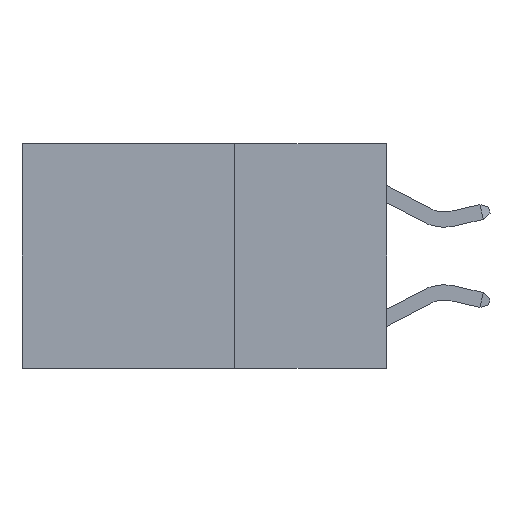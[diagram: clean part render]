
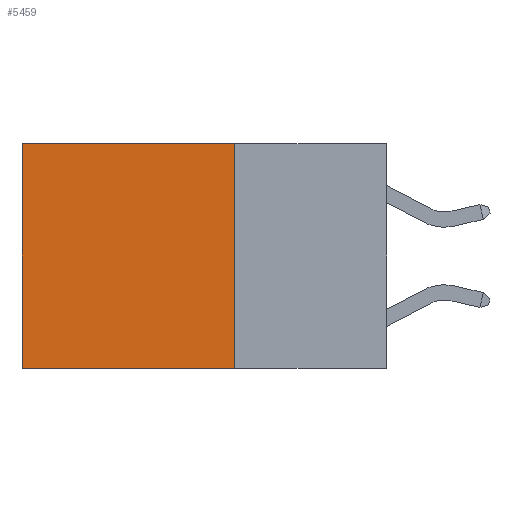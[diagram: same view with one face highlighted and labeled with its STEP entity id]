
A CAD part, left-side view. The second image highlights one B-rep face of the part: STEP entity #5459.
In plain terms, the highlighted planar face has unit normal (-1, 0, 0).
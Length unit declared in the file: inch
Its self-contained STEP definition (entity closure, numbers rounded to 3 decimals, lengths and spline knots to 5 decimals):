
#92 = VECTOR ( 'NONE', #7113, 39.37008 ) ;
#1116 = CARTESIAN_POINT ( 'NONE',  ( 0.2625, 0.25, 0. ) ) ;
#1292 = CARTESIAN_POINT ( 'NONE',  ( 0.2625, 0.25, 0. ) ) ;
#1621 = CARTESIAN_POINT ( 'NONE',  ( 0.2625, 0.25, 0. ) ) ;
#1662 = EDGE_CURVE ( 'NONE', #11066, #3941, #6057, .T. ) ;
#1735 = CARTESIAN_POINT ( 'NONE',  ( 0.2625, 0.6, -0.37 ) ) ;
#2175 = CARTESIAN_POINT ( 'NONE',  ( 0.2625, 0.6, 0. ) ) ;
#2228 = EDGE_CURVE ( 'NONE', #5541, #7366, #2628, .T. ) ;
#2399 = CARTESIAN_POINT ( 'NONE',  ( 0.2625, 0.6, 0. ) ) ;
#2628 = LINE ( 'NONE', #2175, #92 ) ;
#3175 = DIRECTION ( 'NONE',  ( 1., 0., 0. ) ) ;
#3426 = AXIS2_PLACEMENT_3D ( 'NONE', #1292, #3175, #9885 ) ;
#3941 = VERTEX_POINT ( 'NONE', #7762 ) ;
#4006 = VECTOR ( 'NONE', #6964, 39.37008 ) ;
#5459 = ADVANCED_FACE ( 'NONE', ( #7054 ), #8998, .F. ) ;
#5541 = VERTEX_POINT ( 'NONE', #2399 ) ;
#5785 = VECTOR ( 'NONE', #8260, 39.37008 ) ;
#6057 = LINE ( 'NONE', #6936, #5785 ) ;
#6486 = DIRECTION ( 'NONE',  ( 0., 1., 0. ) ) ;
#6805 = EDGE_LOOP ( 'NONE', ( #8060, #11076, #7395, #7443 ) ) ;
#6936 = CARTESIAN_POINT ( 'NONE',  ( 0.2625, 0.25, 0. ) ) ;
#6964 = DIRECTION ( 'NONE',  ( 0., 1., 0. ) ) ;
#7054 = FACE_OUTER_BOUND ( 'NONE', #6805, .T. ) ;
#7113 = DIRECTION ( 'NONE',  ( 0., 0., -1. ) ) ;
#7366 = VERTEX_POINT ( 'NONE', #1735 ) ;
#7395 = ORIENTED_EDGE ( 'NONE', *, *, #1662, .F. ) ;
#7443 = ORIENTED_EDGE ( 'NONE', *, *, #11663, .T. ) ;
#7762 = CARTESIAN_POINT ( 'NONE',  ( 0.2625, 0.25, -0.37 ) ) ;
#8060 = ORIENTED_EDGE ( 'NONE', *, *, #2228, .T. ) ;
#8260 = DIRECTION ( 'NONE',  ( 0., 0., -1. ) ) ;
#8998 = PLANE ( 'NONE',  #3426 ) ;
#9297 = EDGE_CURVE ( 'NONE', #3941, #7366, #11479, .T. ) ;
#9417 = LINE ( 'NONE', #1621, #11725 ) ;
#9885 = DIRECTION ( 'NONE',  ( 0., 0., -1. ) ) ;
#11066 = VERTEX_POINT ( 'NONE', #1116 ) ;
#11076 = ORIENTED_EDGE ( 'NONE', *, *, #9297, .F. ) ;
#11446 = CARTESIAN_POINT ( 'NONE',  ( 0.2625, 0.25, -0.37 ) ) ;
#11479 = LINE ( 'NONE', #11446, #4006 ) ;
#11663 = EDGE_CURVE ( 'NONE', #11066, #5541, #9417, .T. ) ;
#11725 = VECTOR ( 'NONE', #6486, 39.37008 ) ;
